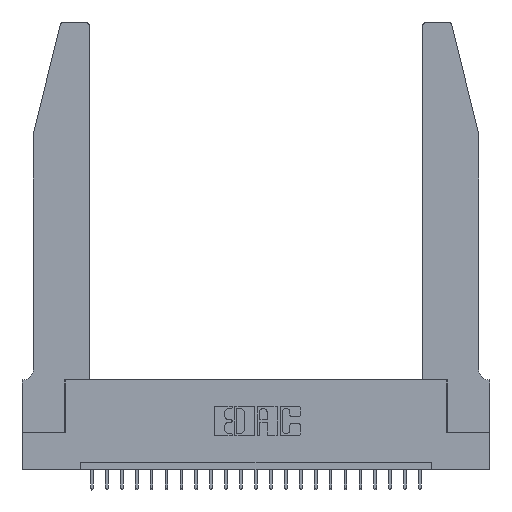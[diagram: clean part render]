
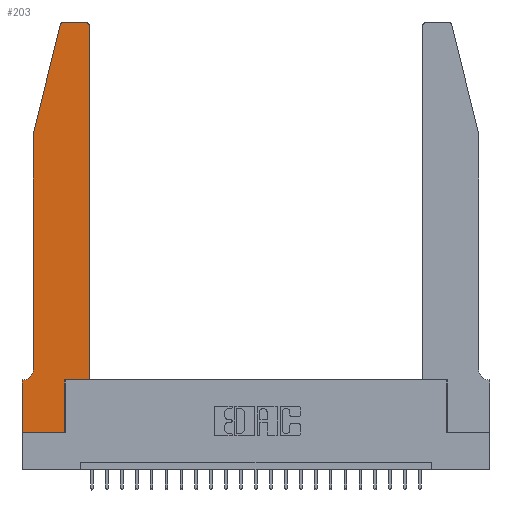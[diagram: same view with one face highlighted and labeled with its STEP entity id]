
A CAD part, top view. The second image highlights one B-rep face of the part: STEP entity #203.
In plain terms, the highlighted planar face has unit normal (0, 0, 1).
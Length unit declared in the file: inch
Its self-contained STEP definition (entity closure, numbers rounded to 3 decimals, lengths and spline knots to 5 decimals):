
#203 = ADVANCED_FACE ( 'NONE', ( #8728 ), #16377, .T. ) ;
#210 = CARTESIAN_POINT ( 'NONE',  ( 0., 0., 0.37 ) ) ;
#375 = CARTESIAN_POINT ( 'NONE',  ( 0.4505, 2.72, 0.37 ) ) ;
#524 = EDGE_CURVE ( 'NONE', #14256, #16754, #990, .T. ) ;
#973 = CARTESIAN_POINT ( 'NONE',  ( 0.284, 2.72, 0.37 ) ) ;
#990 = LINE ( 'NONE', #13378, #17696 ) ;
#1206 = LINE ( 'NONE', #12603, #10880 ) ;
#1232 = LINE ( 'NONE', #1600, #8239 ) ;
#1321 = DIRECTION ( 'NONE',  ( 0., 1., 0. ) ) ;
#1600 = CARTESIAN_POINT ( 'NONE',  ( 0.0755, 0.35, 0.37 ) ) ;
#1671 = EDGE_CURVE ( 'NONE', #3257, #5785, #8896, .T. ) ;
#1727 = VECTOR ( 'NONE', #21830, 39.37008 ) ;
#1887 = VERTEX_POINT ( 'NONE', #18306 ) ;
#1950 = CARTESIAN_POINT ( 'NONE',  ( 0.0055, 0.42, 0.37 ) ) ;
#2230 = EDGE_CURVE ( 'NONE', #24057, #22960, #23466, .T. ) ;
#2673 = ORIENTED_EDGE ( 'NONE', *, *, #1671, .T. ) ;
#3257 = VERTEX_POINT ( 'NONE', #6022 ) ;
#3636 = DIRECTION ( 'NONE',  ( 1., 0., 0. ) ) ;
#3701 = EDGE_CURVE ( 'NONE', #13593, #10452, #4351, .T. ) ;
#3706 = DIRECTION ( 'NONE',  ( 1., 0., 0. ) ) ;
#4351 = LINE ( 'NONE', #19743, #19761 ) ;
#5255 = LINE ( 'NONE', #24553, #24297 ) ;
#5556 = EDGE_CURVE ( 'NONE', #5785, #24057, #1232, .T. ) ;
#5704 = EDGE_CURVE ( 'NONE', #6731, #13593, #16277, .T. ) ;
#5785 = VERTEX_POINT ( 'NONE', #9072 ) ;
#6022 = CARTESIAN_POINT ( 'NONE',  ( 0.0755, 0.42, 0.37 ) ) ;
#6193 = EDGE_CURVE ( 'NONE', #1887, #14256, #8621, .T. ) ;
#6324 = CARTESIAN_POINT ( 'NONE',  ( 0., 0., 0.37 ) ) ;
#6358 = CIRCLE ( 'NONE', #20323, 0.03 ) ;
#6731 = VERTEX_POINT ( 'NONE', #12120 ) ;
#6828 = DIRECTION ( 'NONE',  ( 1., 0., 0. ) ) ;
#7429 = AXIS2_PLACEMENT_3D ( 'NONE', #973, #8588, #16254 ) ;
#7809 = DIRECTION ( 'NONE',  ( 1., 0., 0. ) ) ;
#7957 = VERTEX_POINT ( 'NONE', #375 ) ;
#8051 = EDGE_CURVE ( 'NONE', #11524, #6731, #5255, .T. ) ;
#8067 = LINE ( 'NONE', #17431, #17680 ) ;
#8239 = VECTOR ( 'NONE', #9218, 39.37008 ) ;
#8384 = ORIENTED_EDGE ( 'NONE', *, *, #22563, .T. ) ;
#8588 = DIRECTION ( 'NONE',  ( 0., 0., 1. ) ) ;
#8621 = LINE ( 'NONE', #18371, #12675 ) ;
#8728 = FACE_OUTER_BOUND ( 'NONE', #23721, .T. ) ;
#8896 = CIRCLE ( 'NONE', #12571, 0.07 ) ;
#9072 = CARTESIAN_POINT ( 'NONE',  ( 0.0055, 0.35, 0.37 ) ) ;
#9154 = DIRECTION ( 'NONE',  ( -1., 0., 0. ) ) ;
#9218 = DIRECTION ( 'NONE',  ( -1., 0., 0. ) ) ;
#9223 = ORIENTED_EDGE ( 'NONE', *, *, #6193, .T. ) ;
#9225 = EDGE_CURVE ( 'NONE', #16754, #7957, #1206, .T. ) ;
#9411 = EDGE_CURVE ( 'NONE', #22960, #1887, #17310, .T. ) ;
#9560 = DIRECTION ( 'NONE',  ( 0., 0., -1. ) ) ;
#9988 = DIRECTION ( 'NONE',  ( -0.239, -0.971, 0. ) ) ;
#9991 = ORIENTED_EDGE ( 'NONE', *, *, #524, .T. ) ;
#10452 = VERTEX_POINT ( 'NONE', #17186 ) ;
#10880 = VECTOR ( 'NONE', #1321, 39.37008 ) ;
#11524 = VERTEX_POINT ( 'NONE', #13311 ) ;
#11549 = ORIENTED_EDGE ( 'NONE', *, *, #12014, .T. ) ;
#12014 = EDGE_CURVE ( 'NONE', #10452, #3257, #8067, .T. ) ;
#12120 = CARTESIAN_POINT ( 'NONE',  ( 0.284, 2.75, 0.37 ) ) ;
#12571 = AXIS2_PLACEMENT_3D ( 'NONE', #1950, #9560, #21331 ) ;
#12603 = CARTESIAN_POINT ( 'NONE',  ( 0.4505, 0.35, 0.37 ) ) ;
#12675 = VECTOR ( 'NONE', #20112, 39.37008 ) ;
#12809 = DIRECTION ( 'NONE',  ( 0., 0., 1. ) ) ;
#13311 = CARTESIAN_POINT ( 'NONE',  ( 0.4205, 2.75, 0.37 ) ) ;
#13378 = CARTESIAN_POINT ( 'NONE',  ( 0.4505, 0.35, 0.37 ) ) ;
#13593 = VERTEX_POINT ( 'NONE', #22210 ) ;
#14256 = VERTEX_POINT ( 'NONE', #16330 ) ;
#14816 = ORIENTED_EDGE ( 'NONE', *, *, #3701, .T. ) ;
#15239 = ORIENTED_EDGE ( 'NONE', *, *, #5556, .T. ) ;
#15600 = DIRECTION ( 'NONE',  ( 0., -1., 0. ) ) ;
#16254 = DIRECTION ( 'NONE',  ( 1., 0., 0. ) ) ;
#16277 = CIRCLE ( 'NONE', #7429, 0.03 ) ;
#16330 = CARTESIAN_POINT ( 'NONE',  ( 0.2865, 0.35, 0.37 ) ) ;
#16377 = PLANE ( 'NONE',  #19716 ) ;
#16754 = VERTEX_POINT ( 'NONE', #21505 ) ;
#17186 = CARTESIAN_POINT ( 'NONE',  ( 0.0755, 2., 0.37 ) ) ;
#17310 = LINE ( 'NONE', #210, #20438 ) ;
#17431 = CARTESIAN_POINT ( 'NONE',  ( 0.0755, 2., 0.37 ) ) ;
#17680 = VECTOR ( 'NONE', #15600, 39.37008 ) ;
#17696 = VECTOR ( 'NONE', #3706, 39.37008 ) ;
#18073 = ORIENTED_EDGE ( 'NONE', *, *, #8051, .T. ) ;
#18306 = CARTESIAN_POINT ( 'NONE',  ( 0.2865, 0., 0.37 ) ) ;
#18371 = CARTESIAN_POINT ( 'NONE',  ( 0.2865, 0.35, 0.37 ) ) ;
#19606 = DIRECTION ( 'NONE',  ( 0., 0., 1. ) ) ;
#19632 = ORIENTED_EDGE ( 'NONE', *, *, #2230, .T. ) ;
#19716 = AXIS2_PLACEMENT_3D ( 'NONE', #23970, #19606, #6828 ) ;
#19743 = CARTESIAN_POINT ( 'NONE',  ( 0.0755, 2., 0.37 ) ) ;
#19761 = VECTOR ( 'NONE', #9988, 39.37008 ) ;
#20112 = DIRECTION ( 'NONE',  ( 0., 1., 0. ) ) ;
#20323 = AXIS2_PLACEMENT_3D ( 'NONE', #24656, #12809, #3636 ) ;
#20438 = VECTOR ( 'NONE', #7809, 39.37008 ) ;
#21085 = CARTESIAN_POINT ( 'NONE',  ( 0., 0.35, 0.37 ) ) ;
#21331 = DIRECTION ( 'NONE',  ( -1., 0., 0. ) ) ;
#21505 = CARTESIAN_POINT ( 'NONE',  ( 0.4505, 0.35, 0.37 ) ) ;
#21737 = CARTESIAN_POINT ( 'NONE',  ( 0., 0., 0.37 ) ) ;
#21830 = DIRECTION ( 'NONE',  ( 0., -1., 0. ) ) ;
#22132 = ORIENTED_EDGE ( 'NONE', *, *, #5704, .T. ) ;
#22210 = CARTESIAN_POINT ( 'NONE',  ( 0.25487, 2.72718, 0.37 ) ) ;
#22563 = EDGE_CURVE ( 'NONE', #7957, #11524, #6358, .T. ) ;
#22960 = VERTEX_POINT ( 'NONE', #21737 ) ;
#23466 = LINE ( 'NONE', #6324, #1727 ) ;
#23657 = ORIENTED_EDGE ( 'NONE', *, *, #9225, .T. ) ;
#23659 = ORIENTED_EDGE ( 'NONE', *, *, #9411, .T. ) ;
#23721 = EDGE_LOOP ( 'NONE', ( #18073, #22132, #14816, #11549, #2673, #15239, #19632, #23659, #9223, #9991, #23657, #8384 ) ) ;
#23970 = CARTESIAN_POINT ( 'NONE',  ( 0., 0.35, 0.37 ) ) ;
#24057 = VERTEX_POINT ( 'NONE', #21085 ) ;
#24297 = VECTOR ( 'NONE', #9154, 39.37008 ) ;
#24553 = CARTESIAN_POINT ( 'NONE',  ( 0.2605, 2.75, 0.37 ) ) ;
#24656 = CARTESIAN_POINT ( 'NONE',  ( 0.4205, 2.72, 0.37 ) ) ;
